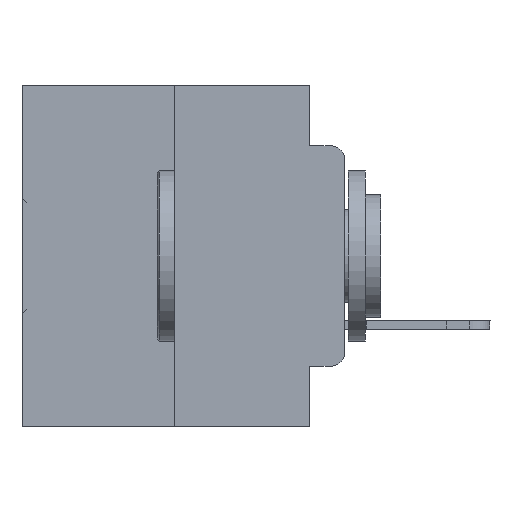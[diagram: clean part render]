
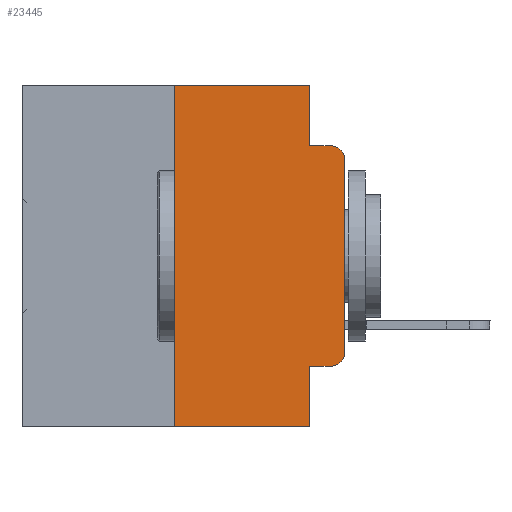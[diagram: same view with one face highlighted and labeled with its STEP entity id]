
A CAD part, left-side view. The second image highlights one B-rep face of the part: STEP entity #23445.
In plain terms, the highlighted planar face has unit normal (-1, 0, 0).
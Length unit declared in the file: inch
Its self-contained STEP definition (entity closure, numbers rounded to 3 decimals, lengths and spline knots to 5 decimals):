
#845 = EDGE_CURVE ( 'NONE', #18319, #18105, #20857, .T. ) ;
#941 = CARTESIAN_POINT ( 'NONE',  ( 0., 0.25, -0.5 ) ) ;
#1406 = AXIS2_PLACEMENT_3D ( 'NONE', #20200, #1936, #4606 ) ;
#1661 = EDGE_CURVE ( 'NONE', #33922, #18319, #29872, .T. ) ;
#1682 = VECTOR ( 'NONE', #11189, 39.37008 ) ;
#1936 = DIRECTION ( 'NONE',  ( -1., 0., 0. ) ) ;
#2655 = LINE ( 'NONE', #23877, #17150 ) ;
#2706 = ORIENTED_EDGE ( 'NONE', *, *, #22750, .F. ) ;
#2747 = LINE ( 'NONE', #26016, #24598 ) ;
#3498 = CARTESIAN_POINT ( 'NONE',  ( 0., 0.473, -0.5 ) ) ;
#4606 = DIRECTION ( 'NONE',  ( 0., 0., -1. ) ) ;
#5220 = CARTESIAN_POINT ( 'NONE',  ( 0., 0.473, 0. ) ) ;
#5329 = PLANE ( 'NONE',  #33620 ) ;
#5544 = CIRCLE ( 'NONE', #16569, 0.02 ) ;
#5805 = LINE ( 'NONE', #7534, #1682 ) ;
#6650 = CARTESIAN_POINT ( 'NONE',  ( 0., 0.051, 0. ) ) ;
#6709 = EDGE_CURVE ( 'NONE', #33922, #17431, #29524, .T. ) ;
#6810 = VECTOR ( 'NONE', #7993, 39.37008 ) ;
#7534 = CARTESIAN_POINT ( 'NONE',  ( 0., 0.051, -0.4115 ) ) ;
#7565 = CARTESIAN_POINT ( 'NONE',  ( 0., 0.051, -0.0885 ) ) ;
#7896 = DIRECTION ( 'NONE',  ( 0., 0., 1. ) ) ;
#7993 = DIRECTION ( 'NONE',  ( 0., -1., 0. ) ) ;
#8035 = CARTESIAN_POINT ( 'NONE',  ( 0., 0.02, -0.0885 ) ) ;
#9103 = ORIENTED_EDGE ( 'NONE', *, *, #19520, .F. ) ;
#9374 = VERTEX_POINT ( 'NONE', #7565 ) ;
#9507 = DIRECTION ( 'NONE',  ( 0., 0., -1. ) ) ;
#9813 = CARTESIAN_POINT ( 'NONE',  ( 0., 0., 0. ) ) ;
#10376 = EDGE_LOOP ( 'NONE', ( #11713, #16453, #9103, #2706, #27981, #19798, #19208, #27265, #28303, #33695 ) ) ;
#10672 = DIRECTION ( 'NONE',  ( 1., 0., 0. ) ) ;
#11189 = DIRECTION ( 'NONE',  ( 0., -1., 0. ) ) ;
#11713 = ORIENTED_EDGE ( 'NONE', *, *, #26269, .T. ) ;
#12144 = VERTEX_POINT ( 'NONE', #27357 ) ;
#13090 = EDGE_CURVE ( 'NONE', #12144, #20734, #13432, .T. ) ;
#13432 = CIRCLE ( 'NONE', #1406, 0.02 ) ;
#14590 = DIRECTION ( 'NONE',  ( -1., 0., 0. ) ) ;
#14895 = LINE ( 'NONE', #19551, #17383 ) ;
#15079 = DIRECTION ( 'NONE',  ( 0., -1., 0. ) ) ;
#15243 = CARTESIAN_POINT ( 'NONE',  ( 0., 0.051, -0.5 ) ) ;
#15675 = CARTESIAN_POINT ( 'NONE',  ( 0., 0.25, 0. ) ) ;
#15836 = CARTESIAN_POINT ( 'NONE',  ( 0., 0.473, 0. ) ) ;
#16007 = VERTEX_POINT ( 'NONE', #17602 ) ;
#16453 = ORIENTED_EDGE ( 'NONE', *, *, #13090, .T. ) ;
#16569 = AXIS2_PLACEMENT_3D ( 'NONE', #17604, #14590, #9507 ) ;
#16701 = VECTOR ( 'NONE', #25355, 39.37008 ) ;
#17150 = VECTOR ( 'NONE', #26324, 39.37008 ) ;
#17153 = LINE ( 'NONE', #9813, #16701 ) ;
#17383 = VECTOR ( 'NONE', #30019, 39.37008 ) ;
#17431 = VERTEX_POINT ( 'NONE', #15243 ) ;
#17602 = CARTESIAN_POINT ( 'NONE',  ( 0., 0.051, -0.4115 ) ) ;
#17604 = CARTESIAN_POINT ( 'NONE',  ( 0., 0.02, -0.3915 ) ) ;
#18105 = VERTEX_POINT ( 'NONE', #6650 ) ;
#18207 = CARTESIAN_POINT ( 'NONE',  ( 0., 0.25, 0. ) ) ;
#18297 = CARTESIAN_POINT ( 'NONE',  ( 0., 0.02, -0.4115 ) ) ;
#18319 = VERTEX_POINT ( 'NONE', #15675 ) ;
#19208 = ORIENTED_EDGE ( 'NONE', *, *, #6709, .T. ) ;
#19520 = EDGE_CURVE ( 'NONE', #9374, #20734, #2747, .T. ) ;
#19551 = CARTESIAN_POINT ( 'NONE',  ( 0., 0.051, 0. ) ) ;
#19798 = ORIENTED_EDGE ( 'NONE', *, *, #1661, .F. ) ;
#20200 = CARTESIAN_POINT ( 'NONE',  ( 0., 0.02, -0.1085 ) ) ;
#20734 = VERTEX_POINT ( 'NONE', #8035 ) ;
#20857 = LINE ( 'NONE', #15836, #6810 ) ;
#20914 = EDGE_CURVE ( 'NONE', #25641, #25951, #5544, .T. ) ;
#21226 = EDGE_CURVE ( 'NONE', #16007, #17431, #2655, .T. ) ;
#21952 = DIRECTION ( 'NONE',  ( 0., -1., 0. ) ) ;
#22505 = VECTOR ( 'NONE', #21952, 39.37008 ) ;
#22750 = EDGE_CURVE ( 'NONE', #18105, #9374, #14895, .T. ) ;
#23445 = ADVANCED_FACE ( 'NONE', ( #32096 ), #5329, .F. ) ;
#23877 = CARTESIAN_POINT ( 'NONE',  ( 0., 0.051, 0. ) ) ;
#24598 = VECTOR ( 'NONE', #15079, 39.37008 ) ;
#25355 = DIRECTION ( 'NONE',  ( 0., 0., 1. ) ) ;
#25641 = VERTEX_POINT ( 'NONE', #18297 ) ;
#25951 = VERTEX_POINT ( 'NONE', #32643 ) ;
#26016 = CARTESIAN_POINT ( 'NONE',  ( 0., 0.051, -0.0885 ) ) ;
#26269 = EDGE_CURVE ( 'NONE', #25951, #12144, #17153, .T. ) ;
#26324 = DIRECTION ( 'NONE',  ( 0., 0., -1. ) ) ;
#26565 = VECTOR ( 'NONE', #7896, 39.37008 ) ;
#27265 = ORIENTED_EDGE ( 'NONE', *, *, #21226, .F. ) ;
#27357 = CARTESIAN_POINT ( 'NONE',  ( 0., 0., -0.1085 ) ) ;
#27859 = EDGE_CURVE ( 'NONE', #16007, #25641, #5805, .T. ) ;
#27981 = ORIENTED_EDGE ( 'NONE', *, *, #845, .F. ) ;
#28303 = ORIENTED_EDGE ( 'NONE', *, *, #27859, .T. ) ;
#29524 = LINE ( 'NONE', #3498, #22505 ) ;
#29872 = LINE ( 'NONE', #18207, #26565 ) ;
#30019 = DIRECTION ( 'NONE',  ( 0., 0., -1. ) ) ;
#31729 = DIRECTION ( 'NONE',  ( 0., 0., -1. ) ) ;
#32096 = FACE_OUTER_BOUND ( 'NONE', #10376, .T. ) ;
#32643 = CARTESIAN_POINT ( 'NONE',  ( 0., 0., -0.3915 ) ) ;
#33620 = AXIS2_PLACEMENT_3D ( 'NONE', #5220, #10672, #31729 ) ;
#33695 = ORIENTED_EDGE ( 'NONE', *, *, #20914, .T. ) ;
#33922 = VERTEX_POINT ( 'NONE', #941 ) ;
